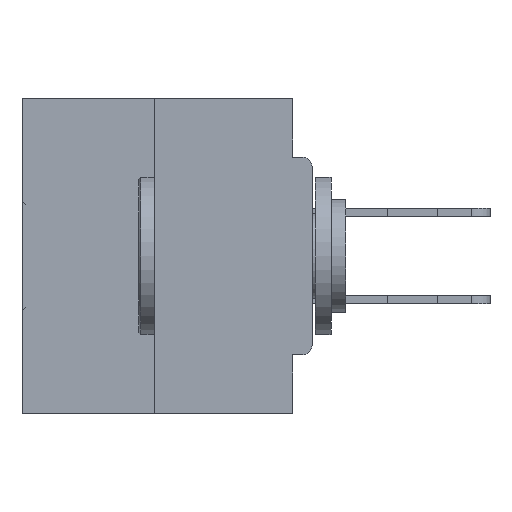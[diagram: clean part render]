
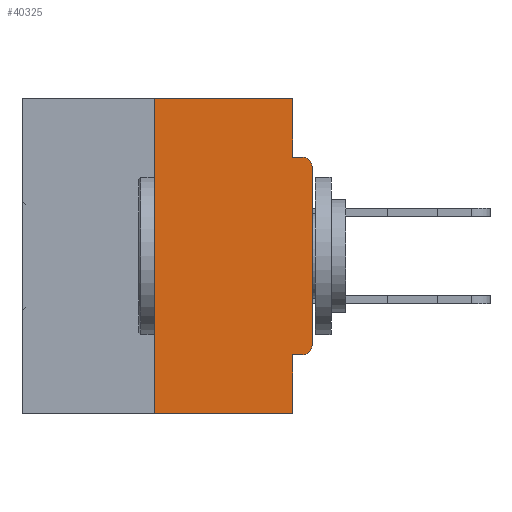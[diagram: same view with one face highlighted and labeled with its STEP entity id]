
A CAD part, left-side view. The second image highlights one B-rep face of the part: STEP entity #40325.
In plain terms, the highlighted planar face has unit normal (-1, 0, 0).
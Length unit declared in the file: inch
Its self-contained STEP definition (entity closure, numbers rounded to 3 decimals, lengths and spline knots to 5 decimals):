
#15 = VERTEX_POINT ( 'NONE', #6322 ) ;
#681 = LINE ( 'NONE', #12446, #14366 ) ;
#1368 = LINE ( 'NONE', #3739, #24029 ) ;
#1854 = VECTOR ( 'NONE', #22135, 39.37008 ) ;
#1938 = VECTOR ( 'NONE', #29719, 39.37008 ) ;
#2808 = VERTEX_POINT ( 'NONE', #30925 ) ;
#3119 = DIRECTION ( 'NONE',  ( 0., -1., 0. ) ) ;
#3224 = CARTESIAN_POINT ( 'NONE',  ( 0., 0., -0.0935 ) ) ;
#3739 = CARTESIAN_POINT ( 'NONE',  ( 0., 0.031, -0.5 ) ) ;
#4800 = LINE ( 'NONE', #19743, #22147 ) ;
#5815 = PLANE ( 'NONE',  #27643 ) ;
#5951 = CARTESIAN_POINT ( 'NONE',  ( 0., 0.46, -0.5 ) ) ;
#6039 = ORIENTED_EDGE ( 'NONE', *, *, #23628, .T. ) ;
#6322 = CARTESIAN_POINT ( 'NONE',  ( 0., 0., -0.3915 ) ) ;
#6524 = DIRECTION ( 'NONE',  ( 0., 0., -1. ) ) ;
#7152 = DIRECTION ( 'NONE',  ( 0., 0., -1. ) ) ;
#10072 = CARTESIAN_POINT ( 'NONE',  ( 0., 0., 0. ) ) ;
#10634 = DIRECTION ( 'NONE',  ( 0., 0., -1. ) ) ;
#12141 = VERTEX_POINT ( 'NONE', #30716 ) ;
#12292 = DIRECTION ( 'NONE',  ( 0., 0., 1. ) ) ;
#12309 = VERTEX_POINT ( 'NONE', #21958 ) ;
#12446 = CARTESIAN_POINT ( 'NONE',  ( 0., 0.25, 0. ) ) ;
#12465 = VERTEX_POINT ( 'NONE', #13625 ) ;
#13374 = CARTESIAN_POINT ( 'NONE',  ( 0., 0.015, -0.1085 ) ) ;
#13488 = CIRCLE ( 'NONE', #40377, 0.015 ) ;
#13625 = CARTESIAN_POINT ( 'NONE',  ( 0., 0.015, -0.4065 ) ) ;
#14001 = LINE ( 'NONE', #31250, #23499 ) ;
#14117 = CARTESIAN_POINT ( 'NONE',  ( 0., 0.031, -0.0935 ) ) ;
#14366 = VECTOR ( 'NONE', #12292, 39.37008 ) ;
#14823 = VERTEX_POINT ( 'NONE', #39064 ) ;
#15699 = VERTEX_POINT ( 'NONE', #27314 ) ;
#15737 = CARTESIAN_POINT ( 'NONE',  ( 0., 0., -0.4065 ) ) ;
#16016 = AXIS2_PLACEMENT_3D ( 'NONE', #13374, #17207, #27229 ) ;
#16486 = DIRECTION ( 'NONE',  ( 1., 0., 0. ) ) ;
#16800 = ORIENTED_EDGE ( 'NONE', *, *, #29075, .T. ) ;
#17207 = DIRECTION ( 'NONE',  ( -1., 0., 0. ) ) ;
#17570 = DIRECTION ( 'NONE',  ( -1., 0., 0. ) ) ;
#18633 = ORIENTED_EDGE ( 'NONE', *, *, #24526, .T. ) ;
#19743 = CARTESIAN_POINT ( 'NONE',  ( 0., 0.46, 0. ) ) ;
#19904 = ORIENTED_EDGE ( 'NONE', *, *, #36741, .F. ) ;
#20725 = ORIENTED_EDGE ( 'NONE', *, *, #36746, .F. ) ;
#20945 = LINE ( 'NONE', #3224, #1938 ) ;
#21958 = CARTESIAN_POINT ( 'NONE',  ( 0., 0.25, -0.5 ) ) ;
#21960 = EDGE_CURVE ( 'NONE', #27961, #14823, #20945, .T. ) ;
#22135 = DIRECTION ( 'NONE',  ( 0., 1., 0. ) ) ;
#22147 = VECTOR ( 'NONE', #3119, 39.37008 ) ;
#22271 = ORIENTED_EDGE ( 'NONE', *, *, #33790, .T. ) ;
#22439 = EDGE_CURVE ( 'NONE', #12309, #24030, #681, .T. ) ;
#22772 = ORIENTED_EDGE ( 'NONE', *, *, #22439, .F. ) ;
#22864 = CARTESIAN_POINT ( 'NONE',  ( 0., 0.25, 0. ) ) ;
#23035 = CARTESIAN_POINT ( 'NONE',  ( 0., 0.46, 0. ) ) ;
#23499 = VECTOR ( 'NONE', #28250, 39.37008 ) ;
#23628 = EDGE_CURVE ( 'NONE', #12465, #15, #13488, .T. ) ;
#24029 = VECTOR ( 'NONE', #10634, 39.37008 ) ;
#24030 = VERTEX_POINT ( 'NONE', #22864 ) ;
#24283 = ORIENTED_EDGE ( 'NONE', *, *, #21960, .F. ) ;
#24526 = EDGE_CURVE ( 'NONE', #12309, #15699, #30811, .T. ) ;
#24578 = ORIENTED_EDGE ( 'NONE', *, *, #26209, .F. ) ;
#26081 = CIRCLE ( 'NONE', #16016, 0.015 ) ;
#26209 = EDGE_CURVE ( 'NONE', #24030, #12141, #4800, .T. ) ;
#27229 = DIRECTION ( 'NONE',  ( 0., 0., -1. ) ) ;
#27314 = CARTESIAN_POINT ( 'NONE',  ( 0., 0.031, -0.5 ) ) ;
#27643 = AXIS2_PLACEMENT_3D ( 'NONE', #23035, #16486, #6524 ) ;
#27961 = VERTEX_POINT ( 'NONE', #14117 ) ;
#28250 = DIRECTION ( 'NONE',  ( 0., 0., -1. ) ) ;
#29075 = EDGE_CURVE ( 'NONE', #15, #39529, #40270, .T. ) ;
#29719 = DIRECTION ( 'NONE',  ( 0., -1., 0. ) ) ;
#30716 = CARTESIAN_POINT ( 'NONE',  ( 0., 0.031, 0. ) ) ;
#30811 = LINE ( 'NONE', #5951, #33995 ) ;
#30870 = LINE ( 'NONE', #15737, #1854 ) ;
#30925 = CARTESIAN_POINT ( 'NONE',  ( 0., 0.031, -0.4065 ) ) ;
#31183 = ORIENTED_EDGE ( 'NONE', *, *, #33566, .F. ) ;
#31250 = CARTESIAN_POINT ( 'NONE',  ( 0., 0.031, 0. ) ) ;
#31808 = VECTOR ( 'NONE', #33679, 39.37008 ) ;
#33566 = EDGE_CURVE ( 'NONE', #12465, #2808, #30870, .T. ) ;
#33679 = DIRECTION ( 'NONE',  ( 0., 0., 1. ) ) ;
#33790 = EDGE_CURVE ( 'NONE', #39529, #14823, #26081, .T. ) ;
#33995 = VECTOR ( 'NONE', #36150, 39.37008 ) ;
#36150 = DIRECTION ( 'NONE',  ( 0., -1., 0. ) ) ;
#36741 = EDGE_CURVE ( 'NONE', #2808, #15699, #1368, .T. ) ;
#36746 = EDGE_CURVE ( 'NONE', #12141, #27961, #14001, .T. ) ;
#38542 = FACE_OUTER_BOUND ( 'NONE', #42695, .T. ) ;
#39058 = CARTESIAN_POINT ( 'NONE',  ( 0., 0., -0.1085 ) ) ;
#39064 = CARTESIAN_POINT ( 'NONE',  ( 0., 0.015, -0.0935 ) ) ;
#39529 = VERTEX_POINT ( 'NONE', #39058 ) ;
#40270 = LINE ( 'NONE', #10072, #31808 ) ;
#40325 = ADVANCED_FACE ( 'NONE', ( #38542 ), #5815, .F. ) ;
#40377 = AXIS2_PLACEMENT_3D ( 'NONE', #41097, #17570, #7152 ) ;
#41097 = CARTESIAN_POINT ( 'NONE',  ( 0., 0.015, -0.3915 ) ) ;
#42695 = EDGE_LOOP ( 'NONE', ( #24578, #22772, #18633, #19904, #31183, #6039, #16800, #22271, #24283, #20725 ) ) ;
